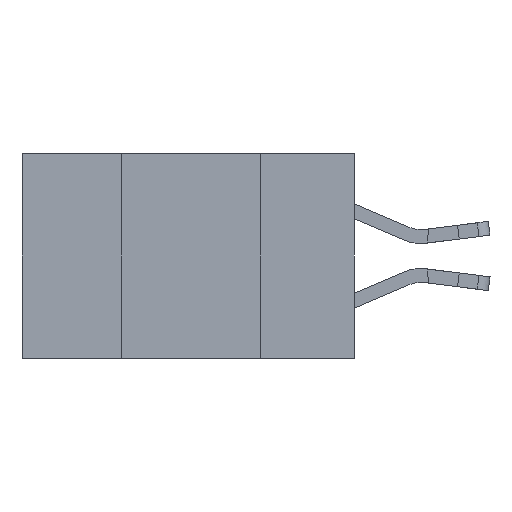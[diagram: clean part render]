
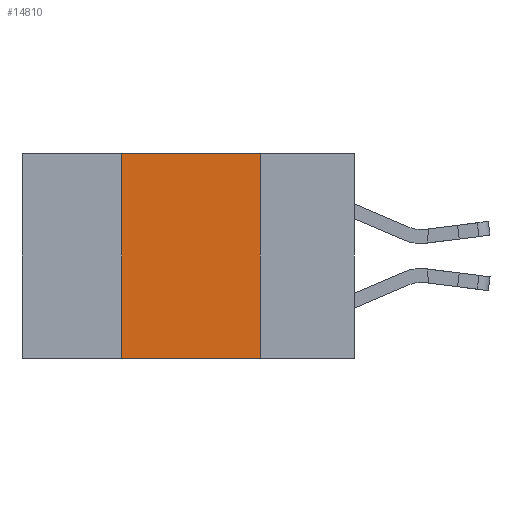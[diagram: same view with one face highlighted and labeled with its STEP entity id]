
A CAD part, left-side view. The second image highlights one B-rep face of the part: STEP entity #14810.
In plain terms, the highlighted planar face has unit normal (-1, 0, 0).
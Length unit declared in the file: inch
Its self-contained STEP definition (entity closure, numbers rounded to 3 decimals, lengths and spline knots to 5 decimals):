
#117 = DIRECTION ( 'NONE',  ( 0., 0., -1. ) ) ;
#788 = VECTOR ( 'NONE', #14512, 39.37008 ) ;
#1070 = CARTESIAN_POINT ( 'NONE',  ( 0., 0.42, 0. ) ) ;
#1378 = EDGE_CURVE ( 'NONE', #10657, #14644, #8601, .T. ) ;
#1458 = EDGE_CURVE ( 'NONE', #5268, #14562, #6426, .T. ) ;
#1718 = CARTESIAN_POINT ( 'NONE',  ( 0., 0.42, 0. ) ) ;
#2068 = ORIENTED_EDGE ( 'NONE', *, *, #14290, .F. ) ;
#2472 = ORIENTED_EDGE ( 'NONE', *, *, #9622, .T. ) ;
#2499 = CARTESIAN_POINT ( 'NONE',  ( 0., 0.17, -0.37 ) ) ;
#3993 = AXIS2_PLACEMENT_3D ( 'NONE', #6263, #14344, #7402 ) ;
#4006 = FACE_OUTER_BOUND ( 'NONE', #8929, .T. ) ;
#4024 = VECTOR ( 'NONE', #5022, 39.37008 ) ;
#4863 = DIRECTION ( 'NONE',  ( 0., -1., 0. ) ) ;
#5022 = DIRECTION ( 'NONE',  ( 0., -1., 0. ) ) ;
#5268 = VERTEX_POINT ( 'NONE', #10217 ) ;
#6263 = CARTESIAN_POINT ( 'NONE',  ( 0., 0.6, 0. ) ) ;
#6426 = LINE ( 'NONE', #1718, #788 ) ;
#6916 = CARTESIAN_POINT ( 'NONE',  ( 0., 0.17, 0. ) ) ;
#7402 = DIRECTION ( 'NONE',  ( 0., 0., -1. ) ) ;
#8558 = LINE ( 'NONE', #14224, #13976 ) ;
#8601 = LINE ( 'NONE', #6916, #10059 ) ;
#8929 = EDGE_LOOP ( 'NONE', ( #10808, #2068, #13937, #2472 ) ) ;
#9088 = LINE ( 'NONE', #14119, #4024 ) ;
#9284 = CARTESIAN_POINT ( 'NONE',  ( 0., 0.17, 0. ) ) ;
#9622 = EDGE_CURVE ( 'NONE', #5268, #14644, #8558, .T. ) ;
#10059 = VECTOR ( 'NONE', #117, 39.37008 ) ;
#10217 = CARTESIAN_POINT ( 'NONE',  ( 0., 0.42, -0.37 ) ) ;
#10657 = VERTEX_POINT ( 'NONE', #9284 ) ;
#10808 = ORIENTED_EDGE ( 'NONE', *, *, #1378, .F. ) ;
#13188 = PLANE ( 'NONE',  #3993 ) ;
#13937 = ORIENTED_EDGE ( 'NONE', *, *, #1458, .F. ) ;
#13976 = VECTOR ( 'NONE', #4863, 39.37008 ) ;
#14119 = CARTESIAN_POINT ( 'NONE',  ( 0., 0.6, 0. ) ) ;
#14224 = CARTESIAN_POINT ( 'NONE',  ( 0., 0.6, -0.37 ) ) ;
#14290 = EDGE_CURVE ( 'NONE', #14562, #10657, #9088, .T. ) ;
#14344 = DIRECTION ( 'NONE',  ( 1., 0., 0. ) ) ;
#14512 = DIRECTION ( 'NONE',  ( 0., 0., 1. ) ) ;
#14562 = VERTEX_POINT ( 'NONE', #1070 ) ;
#14644 = VERTEX_POINT ( 'NONE', #2499 ) ;
#14810 = ADVANCED_FACE ( 'NONE', ( #4006 ), #13188, .F. ) ;
